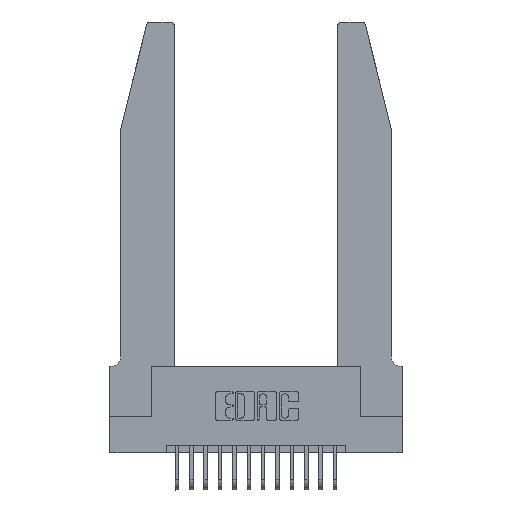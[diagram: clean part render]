
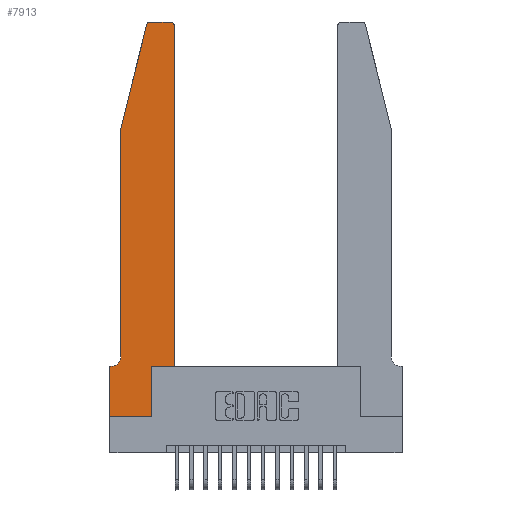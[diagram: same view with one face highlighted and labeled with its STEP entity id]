
A CAD part, top view. The second image highlights one B-rep face of the part: STEP entity #7913.
In plain terms, the highlighted planar face has unit normal (0, 0, 1).
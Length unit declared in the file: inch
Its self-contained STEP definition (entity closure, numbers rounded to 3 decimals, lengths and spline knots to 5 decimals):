
#130 = DIRECTION ( 'NONE',  ( 0., -1., 0. ) ) ;
#281 = VECTOR ( 'NONE', #14039, 39.37008 ) ;
#385 = DIRECTION ( 'NONE',  ( -1., 0., 0. ) ) ;
#483 = CARTESIAN_POINT ( 'NONE',  ( 0.25487, 2.72718, 0.37 ) ) ;
#907 = EDGE_CURVE ( 'NONE', #16656, #3355, #9692, .T. ) ;
#915 = CIRCLE ( 'NONE', #17553, 0.07 ) ;
#957 = CARTESIAN_POINT ( 'NONE',  ( 0.4505, 0.35, 0.37 ) ) ;
#1120 = CARTESIAN_POINT ( 'NONE',  ( 0., 0., 0.37 ) ) ;
#1202 = CIRCLE ( 'NONE', #11796, 0.03 ) ;
#1328 = ORIENTED_EDGE ( 'NONE', *, *, #3711, .T. ) ;
#1753 = LINE ( 'NONE', #9492, #5041 ) ;
#1849 = CARTESIAN_POINT ( 'NONE',  ( 0.4505, 0.35, 0.37 ) ) ;
#1859 = CARTESIAN_POINT ( 'NONE',  ( 0.284, 2.72, 0.37 ) ) ;
#2235 = DIRECTION ( 'NONE',  ( 0., 0., 1. ) ) ;
#2283 = LINE ( 'NONE', #4670, #12467 ) ;
#2286 = ORIENTED_EDGE ( 'NONE', *, *, #15040, .T. ) ;
#2801 = CARTESIAN_POINT ( 'NONE',  ( 0.0755, 2., 0.37 ) ) ;
#2881 = DIRECTION ( 'NONE',  ( 1., 0., 0. ) ) ;
#3100 = ORIENTED_EDGE ( 'NONE', *, *, #10387, .T. ) ;
#3270 = DIRECTION ( 'NONE',  ( 1., 0., 0. ) ) ;
#3290 = DIRECTION ( 'NONE',  ( -1., 0., 0. ) ) ;
#3291 = VECTOR ( 'NONE', #13860, 39.37008 ) ;
#3355 = VERTEX_POINT ( 'NONE', #957 ) ;
#3678 = CARTESIAN_POINT ( 'NONE',  ( 0.0055, 0.35, 0.37 ) ) ;
#3711 = EDGE_CURVE ( 'NONE', #3817, #14590, #915, .T. ) ;
#3817 = VERTEX_POINT ( 'NONE', #10288 ) ;
#4042 = VECTOR ( 'NONE', #130, 39.37008 ) ;
#4253 = DIRECTION ( 'NONE',  ( 0., 0., 1. ) ) ;
#4392 = VERTEX_POINT ( 'NONE', #15172 ) ;
#4473 = LINE ( 'NONE', #16696, #4042 ) ;
#4670 = CARTESIAN_POINT ( 'NONE',  ( 0., 0., 0.37 ) ) ;
#4983 = CARTESIAN_POINT ( 'NONE',  ( 0., 0.35, 0.37 ) ) ;
#4988 = EDGE_CURVE ( 'NONE', #14453, #17529, #5904, .T. ) ;
#5041 = VECTOR ( 'NONE', #10888, 39.37008 ) ;
#5160 = VERTEX_POINT ( 'NONE', #7295 ) ;
#5473 = VECTOR ( 'NONE', #3290, 39.37008 ) ;
#5539 = EDGE_CURVE ( 'NONE', #3355, #14453, #1753, .T. ) ;
#5646 = EDGE_CURVE ( 'NONE', #15069, #4392, #7370, .T. ) ;
#5649 = VERTEX_POINT ( 'NONE', #15215 ) ;
#5899 = LINE ( 'NONE', #8644, #16892 ) ;
#5904 = CIRCLE ( 'NONE', #13466, 0.03 ) ;
#6088 = CARTESIAN_POINT ( 'NONE',  ( 0.4505, 2.72, 0.37 ) ) ;
#6267 = VERTEX_POINT ( 'NONE', #9829 ) ;
#6333 = CARTESIAN_POINT ( 'NONE',  ( 0.2865, 0.35, 0.37 ) ) ;
#6510 = EDGE_LOOP ( 'NONE', ( #3100, #12720, #9022, #15426, #1328, #17217, #10522, #2286, #13131, #15398, #12435, #7985 ) ) ;
#7295 = CARTESIAN_POINT ( 'NONE',  ( 0., 0.35, 0.37 ) ) ;
#7370 = LINE ( 'NONE', #2801, #3291 ) ;
#7913 = ADVANCED_FACE ( 'NONE', ( #10714 ), #10507, .T. ) ;
#7985 = ORIENTED_EDGE ( 'NONE', *, *, #4988, .T. ) ;
#8528 = VERTEX_POINT ( 'NONE', #1120 ) ;
#8644 = CARTESIAN_POINT ( 'NONE',  ( 0.0755, 0.35, 0.37 ) ) ;
#8720 = DIRECTION ( 'NONE',  ( 0., 0., -1. ) ) ;
#9022 = ORIENTED_EDGE ( 'NONE', *, *, #5646, .T. ) ;
#9165 = VECTOR ( 'NONE', #17357, 39.37008 ) ;
#9424 = EDGE_CURVE ( 'NONE', #6267, #16656, #17368, .T. ) ;
#9492 = CARTESIAN_POINT ( 'NONE',  ( 0.4505, 0.35, 0.37 ) ) ;
#9692 = LINE ( 'NONE', #1849, #16573 ) ;
#9829 = CARTESIAN_POINT ( 'NONE',  ( 0.2865, 0., 0.37 ) ) ;
#10288 = CARTESIAN_POINT ( 'NONE',  ( 0.0755, 0.42, 0.37 ) ) ;
#10360 = EDGE_CURVE ( 'NONE', #14590, #5160, #5899, .T. ) ;
#10387 = EDGE_CURVE ( 'NONE', #17529, #5649, #12407, .T. ) ;
#10507 = PLANE ( 'NONE',  #15880 ) ;
#10522 = ORIENTED_EDGE ( 'NONE', *, *, #17071, .T. ) ;
#10714 = FACE_OUTER_BOUND ( 'NONE', #6510, .T. ) ;
#10888 = DIRECTION ( 'NONE',  ( 0., 1., 0. ) ) ;
#11528 = DIRECTION ( 'NONE',  ( 0., 0., 1. ) ) ;
#11544 = CARTESIAN_POINT ( 'NONE',  ( 0.2605, 2.75, 0.37 ) ) ;
#11796 = AXIS2_PLACEMENT_3D ( 'NONE', #1859, #11528, #3270 ) ;
#11913 = DIRECTION ( 'NONE',  ( 1., 0., 0. ) ) ;
#12407 = LINE ( 'NONE', #11544, #5473 ) ;
#12435 = ORIENTED_EDGE ( 'NONE', *, *, #5539, .T. ) ;
#12467 = VECTOR ( 'NONE', #15699, 39.37008 ) ;
#12528 = CARTESIAN_POINT ( 'NONE',  ( 0.4205, 2.72, 0.37 ) ) ;
#12720 = ORIENTED_EDGE ( 'NONE', *, *, #13901, .T. ) ;
#12780 = CARTESIAN_POINT ( 'NONE',  ( 0.2865, 0.35, 0.37 ) ) ;
#12837 = DIRECTION ( 'NONE',  ( -1., 0., 0. ) ) ;
#13131 = ORIENTED_EDGE ( 'NONE', *, *, #9424, .T. ) ;
#13466 = AXIS2_PLACEMENT_3D ( 'NONE', #12528, #4253, #13914 ) ;
#13860 = DIRECTION ( 'NONE',  ( -0.239, -0.971, 0. ) ) ;
#13901 = EDGE_CURVE ( 'NONE', #5649, #15069, #1202, .T. ) ;
#13914 = DIRECTION ( 'NONE',  ( 1., 0., 0. ) ) ;
#14039 = DIRECTION ( 'NONE',  ( 0., -1., 0. ) ) ;
#14453 = VERTEX_POINT ( 'NONE', #6088 ) ;
#14590 = VERTEX_POINT ( 'NONE', #3678 ) ;
#14908 = EDGE_CURVE ( 'NONE', #4392, #3817, #4473, .T. ) ;
#15040 = EDGE_CURVE ( 'NONE', #8528, #6267, #2283, .T. ) ;
#15047 = LINE ( 'NONE', #15403, #281 ) ;
#15069 = VERTEX_POINT ( 'NONE', #483 ) ;
#15172 = CARTESIAN_POINT ( 'NONE',  ( 0.0755, 2., 0.37 ) ) ;
#15215 = CARTESIAN_POINT ( 'NONE',  ( 0.284, 2.75, 0.37 ) ) ;
#15398 = ORIENTED_EDGE ( 'NONE', *, *, #907, .T. ) ;
#15403 = CARTESIAN_POINT ( 'NONE',  ( 0., 0., 0.37 ) ) ;
#15426 = ORIENTED_EDGE ( 'NONE', *, *, #14908, .T. ) ;
#15699 = DIRECTION ( 'NONE',  ( 1., 0., 0. ) ) ;
#15880 = AXIS2_PLACEMENT_3D ( 'NONE', #4983, #2235, #11913 ) ;
#16573 = VECTOR ( 'NONE', #2881, 39.37008 ) ;
#16656 = VERTEX_POINT ( 'NONE', #12780 ) ;
#16696 = CARTESIAN_POINT ( 'NONE',  ( 0.0755, 2., 0.37 ) ) ;
#16892 = VECTOR ( 'NONE', #12837, 39.37008 ) ;
#16979 = CARTESIAN_POINT ( 'NONE',  ( 0.0055, 0.42, 0.37 ) ) ;
#17071 = EDGE_CURVE ( 'NONE', #5160, #8528, #15047, .T. ) ;
#17217 = ORIENTED_EDGE ( 'NONE', *, *, #10360, .T. ) ;
#17357 = DIRECTION ( 'NONE',  ( 0., 1., 0. ) ) ;
#17368 = LINE ( 'NONE', #6333, #9165 ) ;
#17529 = VERTEX_POINT ( 'NONE', #17760 ) ;
#17553 = AXIS2_PLACEMENT_3D ( 'NONE', #16979, #8720, #385 ) ;
#17760 = CARTESIAN_POINT ( 'NONE',  ( 0.4205, 2.75, 0.37 ) ) ;
